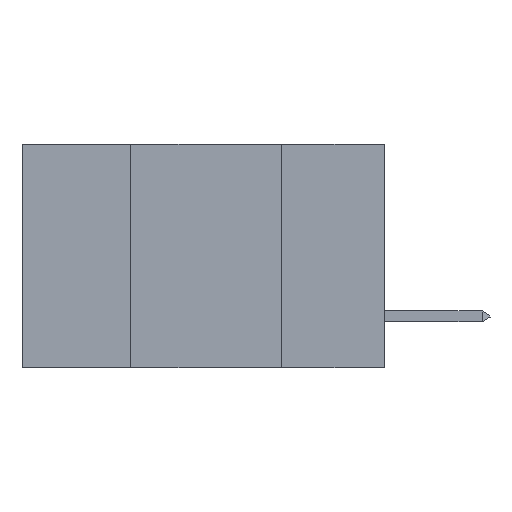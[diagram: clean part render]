
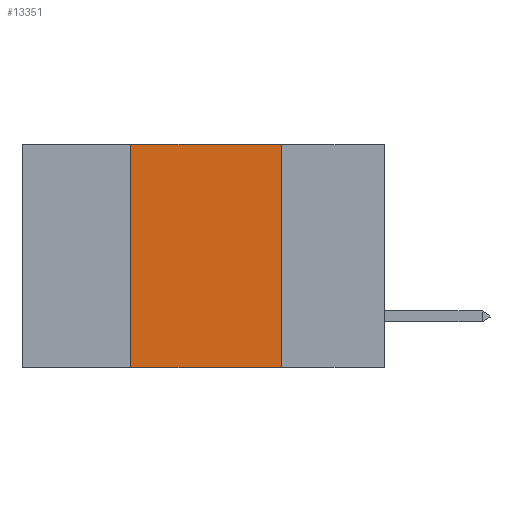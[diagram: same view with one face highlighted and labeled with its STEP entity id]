
A CAD part, left-side view. The second image highlights one B-rep face of the part: STEP entity #13351.
In plain terms, the highlighted planar face has unit normal (-1, 0, 0).
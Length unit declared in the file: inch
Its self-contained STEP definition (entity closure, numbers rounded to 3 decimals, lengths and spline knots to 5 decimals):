
#353 = VECTOR ( 'NONE', #33915, 39.37008 ) ;
#836 = EDGE_CURVE ( 'NONE', #23266, #42412, #21394, .T. ) ;
#3122 = CARTESIAN_POINT ( 'NONE',  ( 0., 0.6, 0. ) ) ;
#4614 = VERTEX_POINT ( 'NONE', #33076 ) ;
#5328 = ORIENTED_EDGE ( 'NONE', *, *, #30933, .F. ) ;
#6318 = LINE ( 'NONE', #15621, #43501 ) ;
#7330 = DIRECTION ( 'NONE',  ( 0., -1., 0. ) ) ;
#7970 = ORIENTED_EDGE ( 'NONE', *, *, #32389, .F. ) ;
#9442 = DIRECTION ( 'NONE',  ( 0., -1., 0. ) ) ;
#13351 = ADVANCED_FACE ( 'NONE', ( #28638 ), #20839, .F. ) ;
#13399 = CARTESIAN_POINT ( 'NONE',  ( 0., 0.6, 0. ) ) ;
#14884 = ORIENTED_EDGE ( 'NONE', *, *, #20143, .F. ) ;
#15621 = CARTESIAN_POINT ( 'NONE',  ( 0., 0.42, 0. ) ) ;
#17258 = VERTEX_POINT ( 'NONE', #36882 ) ;
#20143 = EDGE_CURVE ( 'NONE', #23266, #17258, #6318, .T. ) ;
#20370 = ORIENTED_EDGE ( 'NONE', *, *, #836, .T. ) ;
#20839 = PLANE ( 'NONE',  #31517 ) ;
#21145 = CARTESIAN_POINT ( 'NONE',  ( 0., 0.17, -0.37 ) ) ;
#21394 = LINE ( 'NONE', #21679, #31457 ) ;
#21679 = CARTESIAN_POINT ( 'NONE',  ( 0., 0.6, -0.37 ) ) ;
#22233 = LINE ( 'NONE', #13399, #34042 ) ;
#22378 = LINE ( 'NONE', #34066, #353 ) ;
#23266 = VERTEX_POINT ( 'NONE', #30249 ) ;
#28638 = FACE_OUTER_BOUND ( 'NONE', #32122, .T. ) ;
#30249 = CARTESIAN_POINT ( 'NONE',  ( 0., 0.42, -0.37 ) ) ;
#30933 = EDGE_CURVE ( 'NONE', #4614, #42412, #22378, .T. ) ;
#31457 = VECTOR ( 'NONE', #7330, 39.37008 ) ;
#31517 = AXIS2_PLACEMENT_3D ( 'NONE', #3122, #45984, #35555 ) ;
#32122 = EDGE_LOOP ( 'NONE', ( #5328, #7970, #14884, #20370 ) ) ;
#32389 = EDGE_CURVE ( 'NONE', #17258, #4614, #22233, .T. ) ;
#33076 = CARTESIAN_POINT ( 'NONE',  ( 0., 0.17, 0. ) ) ;
#33915 = DIRECTION ( 'NONE',  ( 0., 0., -1. ) ) ;
#34042 = VECTOR ( 'NONE', #9442, 39.37008 ) ;
#34066 = CARTESIAN_POINT ( 'NONE',  ( 0., 0.17, 0. ) ) ;
#35555 = DIRECTION ( 'NONE',  ( 0., 0., -1. ) ) ;
#36882 = CARTESIAN_POINT ( 'NONE',  ( 0., 0.42, 0. ) ) ;
#42412 = VERTEX_POINT ( 'NONE', #21145 ) ;
#43501 = VECTOR ( 'NONE', #44391, 39.37008 ) ;
#44391 = DIRECTION ( 'NONE',  ( 0., 0., 1. ) ) ;
#45984 = DIRECTION ( 'NONE',  ( 1., 0., 0. ) ) ;
